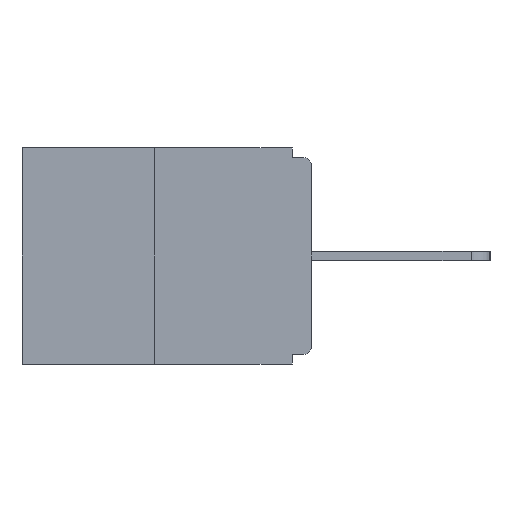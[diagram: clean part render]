
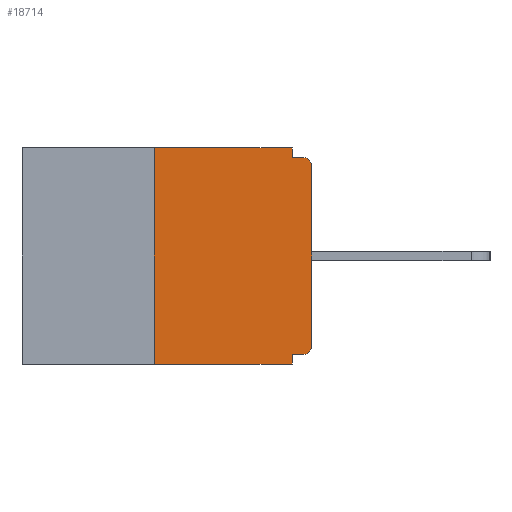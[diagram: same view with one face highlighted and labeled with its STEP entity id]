
A CAD part, left-side view. The second image highlights one B-rep face of the part: STEP entity #18714.
In plain terms, the highlighted planar face has unit normal (-1, 0, 0).
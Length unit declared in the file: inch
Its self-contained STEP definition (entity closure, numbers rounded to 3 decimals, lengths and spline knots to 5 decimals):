
#18 = VERTEX_POINT ( 'NONE', #3237 ) ;
#1569 = EDGE_CURVE ( 'NONE', #11047, #7324, #12752, .T. ) ;
#1671 = DIRECTION ( 'NONE',  ( 0., 0., -1. ) ) ;
#1816 = DIRECTION ( 'NONE',  ( 0., 0., -1. ) ) ;
#1927 = CARTESIAN_POINT ( 'NONE',  ( 0., 0.031, -0.343 ) ) ;
#1949 = LINE ( 'NONE', #7444, #6315 ) ;
#2039 = VERTEX_POINT ( 'NONE', #20227 ) ;
#2884 = DIRECTION ( 'NONE',  ( 0., 0., 1. ) ) ;
#2919 = CARTESIAN_POINT ( 'NONE',  ( 0., 0.015, -0.313 ) ) ;
#3146 = ORIENTED_EDGE ( 'NONE', *, *, #5099, .F. ) ;
#3237 = CARTESIAN_POINT ( 'NONE',  ( 0., 0.25, -0.343 ) ) ;
#3280 = ORIENTED_EDGE ( 'NONE', *, *, #13508, .T. ) ;
#3391 = VERTEX_POINT ( 'NONE', #18779 ) ;
#3692 = CARTESIAN_POINT ( 'NONE',  ( 0., 0.031, 0. ) ) ;
#3772 = CARTESIAN_POINT ( 'NONE',  ( 0., 0.015, -0.03 ) ) ;
#4098 = DIRECTION ( 'NONE',  ( 0., -1., 0. ) ) ;
#4198 = ORIENTED_EDGE ( 'NONE', *, *, #9523, .T. ) ;
#4529 = LINE ( 'NONE', #14469, #11385 ) ;
#5099 = EDGE_CURVE ( 'NONE', #18, #11047, #4529, .T. ) ;
#5116 = DIRECTION ( 'NONE',  ( 0., -1., 0. ) ) ;
#5727 = VERTEX_POINT ( 'NONE', #20249 ) ;
#6286 = CARTESIAN_POINT ( 'NONE',  ( 0., 0.46, 0. ) ) ;
#6315 = VECTOR ( 'NONE', #18928, 39.37008 ) ;
#6613 = EDGE_LOOP ( 'NONE', ( #17156, #3146, #3280, #16276, #7803, #4198, #13218, #17279, #10189, #12524 ) ) ;
#7324 = VERTEX_POINT ( 'NONE', #20924 ) ;
#7444 = CARTESIAN_POINT ( 'NONE',  ( 0., 0., -0.328 ) ) ;
#7803 = ORIENTED_EDGE ( 'NONE', *, *, #18442, .F. ) ;
#7957 = DIRECTION ( 'NONE',  ( 0., 0., -1. ) ) ;
#8728 = DIRECTION ( 'NONE',  ( 0., 0., -1. ) ) ;
#8739 = LINE ( 'NONE', #1927, #19629 ) ;
#8815 = DIRECTION ( 'NONE',  ( -1., 0., 0. ) ) ;
#9081 = AXIS2_PLACEMENT_3D ( 'NONE', #18246, #21436, #13225 ) ;
#9275 = EDGE_CURVE ( 'NONE', #2039, #20748, #8739, .T. ) ;
#9486 = VECTOR ( 'NONE', #4098, 39.37008 ) ;
#9523 = EDGE_CURVE ( 'NONE', #19185, #5727, #11786, .T. ) ;
#9568 = EDGE_CURVE ( 'NONE', #5727, #20664, #18330, .T. ) ;
#9936 = CARTESIAN_POINT ( 'NONE',  ( 0., 0., 0. ) ) ;
#10189 = ORIENTED_EDGE ( 'NONE', *, *, #12642, .F. ) ;
#10801 = EDGE_CURVE ( 'NONE', #7324, #16716, #18572, .T. ) ;
#11047 = VERTEX_POINT ( 'NONE', #18897 ) ;
#11385 = VECTOR ( 'NONE', #2884, 39.37008 ) ;
#11459 = EDGE_CURVE ( 'NONE', #20664, #3391, #20459, .T. ) ;
#11498 = CARTESIAN_POINT ( 'NONE',  ( 0., 0., -0.015 ) ) ;
#11735 = DIRECTION ( 'NONE',  ( 0., -1., 0. ) ) ;
#11786 = CIRCLE ( 'NONE', #14543, 0.015 ) ;
#11802 = VECTOR ( 'NONE', #13105, 39.37008 ) ;
#11954 = LINE ( 'NONE', #13696, #12791 ) ;
#12524 = ORIENTED_EDGE ( 'NONE', *, *, #10801, .F. ) ;
#12642 = EDGE_CURVE ( 'NONE', #16716, #3391, #19813, .T. ) ;
#12752 = LINE ( 'NONE', #6286, #9486 ) ;
#12791 = VECTOR ( 'NONE', #11735, 39.37008 ) ;
#13105 = DIRECTION ( 'NONE',  ( 0., 0., 1. ) ) ;
#13204 = DIRECTION ( 'NONE',  ( -1., 0., 0. ) ) ;
#13218 = ORIENTED_EDGE ( 'NONE', *, *, #9568, .T. ) ;
#13225 = DIRECTION ( 'NONE',  ( 0., 0., -1. ) ) ;
#13508 = EDGE_CURVE ( 'NONE', #18, #20748, #11954, .T. ) ;
#13696 = CARTESIAN_POINT ( 'NONE',  ( 0., 0.46, -0.343 ) ) ;
#14145 = AXIS2_PLACEMENT_3D ( 'NONE', #3772, #8815, #1671 ) ;
#14469 = CARTESIAN_POINT ( 'NONE',  ( 0., 0.25, 0. ) ) ;
#14543 = AXIS2_PLACEMENT_3D ( 'NONE', #2919, #13204, #7957 ) ;
#16276 = ORIENTED_EDGE ( 'NONE', *, *, #9275, .F. ) ;
#16716 = VERTEX_POINT ( 'NONE', #17304 ) ;
#16840 = PLANE ( 'NONE',  #9081 ) ;
#16953 = VECTOR ( 'NONE', #5116, 39.37008 ) ;
#17156 = ORIENTED_EDGE ( 'NONE', *, *, #1569, .F. ) ;
#17175 = CARTESIAN_POINT ( 'NONE',  ( 0., 0.015, -0.328 ) ) ;
#17279 = ORIENTED_EDGE ( 'NONE', *, *, #11459, .T. ) ;
#17304 = CARTESIAN_POINT ( 'NONE',  ( 0., 0.031, -0.015 ) ) ;
#17719 = CARTESIAN_POINT ( 'NONE',  ( 0., 0., -0.03 ) ) ;
#18246 = CARTESIAN_POINT ( 'NONE',  ( 0., 0.46, 0. ) ) ;
#18330 = LINE ( 'NONE', #9936, #11802 ) ;
#18442 = EDGE_CURVE ( 'NONE', #19185, #2039, #1949, .T. ) ;
#18572 = LINE ( 'NONE', #3692, #21485 ) ;
#18714 = ADVANCED_FACE ( 'NONE', ( #20020 ), #16840, .F. ) ;
#18779 = CARTESIAN_POINT ( 'NONE',  ( 0., 0.015, -0.015 ) ) ;
#18897 = CARTESIAN_POINT ( 'NONE',  ( 0., 0.25, 0. ) ) ;
#18928 = DIRECTION ( 'NONE',  ( 0., 1., 0. ) ) ;
#19185 = VERTEX_POINT ( 'NONE', #17175 ) ;
#19629 = VECTOR ( 'NONE', #1816, 39.37008 ) ;
#19813 = LINE ( 'NONE', #11498, #16953 ) ;
#20008 = CARTESIAN_POINT ( 'NONE',  ( 0., 0.031, -0.343 ) ) ;
#20020 = FACE_OUTER_BOUND ( 'NONE', #6613, .T. ) ;
#20227 = CARTESIAN_POINT ( 'NONE',  ( 0., 0.031, -0.328 ) ) ;
#20249 = CARTESIAN_POINT ( 'NONE',  ( 0., 0., -0.313 ) ) ;
#20459 = CIRCLE ( 'NONE', #14145, 0.015 ) ;
#20664 = VERTEX_POINT ( 'NONE', #17719 ) ;
#20748 = VERTEX_POINT ( 'NONE', #20008 ) ;
#20924 = CARTESIAN_POINT ( 'NONE',  ( 0., 0.031, 0. ) ) ;
#21436 = DIRECTION ( 'NONE',  ( 1., 0., 0. ) ) ;
#21485 = VECTOR ( 'NONE', #8728, 39.37008 ) ;
